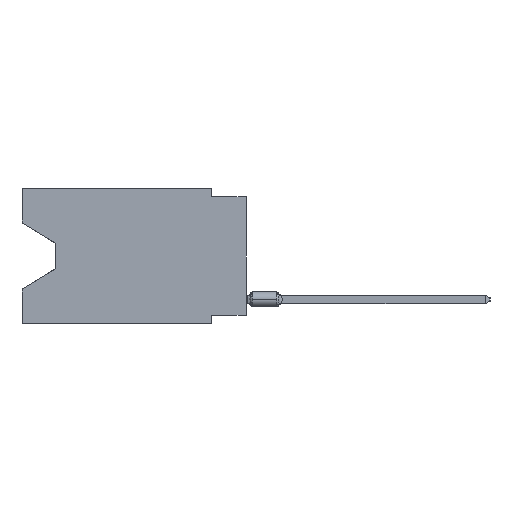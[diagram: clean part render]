
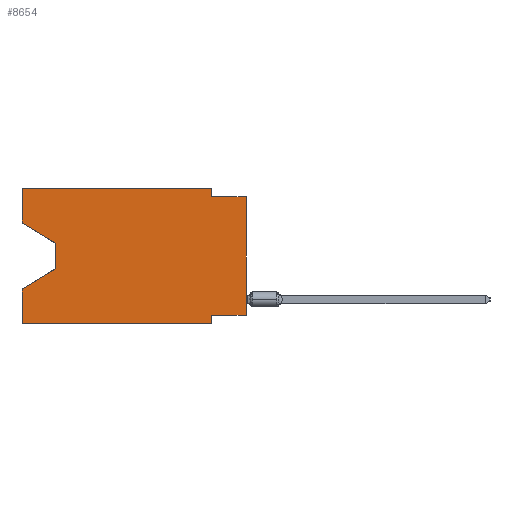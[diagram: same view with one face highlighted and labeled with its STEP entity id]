
A CAD part, left-side view. The second image highlights one B-rep face of the part: STEP entity #8654.
In plain terms, the highlighted planar face has unit normal (-1, 0, 0).
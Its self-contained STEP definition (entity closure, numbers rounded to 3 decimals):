
#57 = VECTOR ( 'NONE', #44217, 1000. ) ;
#443 = EDGE_CURVE ( 'NONE', #57725, #37738, #47207, .T. ) ;
#901 = CARTESIAN_POINT ( 'NONE',  ( 0., 2.54, 0. ) ) ;
#2306 = VERTEX_POINT ( 'NONE', #23278 ) ;
#3446 = DIRECTION ( 'NONE',  ( 0., 0., -1. ) ) ;
#3466 = EDGE_CURVE ( 'NONE', #30836, #67137, #64487, .T. ) ;
#4068 = DIRECTION ( 'NONE',  ( 0., 0., -1. ) ) ;
#4407 = ORIENTED_EDGE ( 'NONE', *, *, #6342, .F. ) ;
#4473 = VECTOR ( 'NONE', #26601, 1000. ) ;
#4868 = VERTEX_POINT ( 'NONE', #29654 ) ;
#5179 = CARTESIAN_POINT ( 'NONE',  ( 0., 0., -9.271 ) ) ;
#6342 = EDGE_CURVE ( 'NONE', #37738, #67137, #57201, .T. ) ;
#7583 = DIRECTION ( 'NONE',  ( 0., -0.855, -0.519 ) ) ;
#8487 = CARTESIAN_POINT ( 'NONE',  ( 0., 16.383, 0. ) ) ;
#8625 = ORIENTED_EDGE ( 'NONE', *, *, #38947, .T. ) ;
#8654 = ADVANCED_FACE ( 'NONE', ( #37394 ), #58468, .F. ) ;
#9928 = EDGE_CURVE ( 'NONE', #51150, #2306, #49291, .T. ) ;
#10958 = DIRECTION ( 'NONE',  ( 0., 1., 0. ) ) ;
#11368 = VECTOR ( 'NONE', #7583, 1000. ) ;
#14093 = CARTESIAN_POINT ( 'NONE',  ( 0., 16.383, -2.546 ) ) ;
#14217 = ORIENTED_EDGE ( 'NONE', *, *, #19808, .F. ) ;
#14324 = CARTESIAN_POINT ( 'NONE',  ( 0., 2.54, -9.906 ) ) ;
#14363 = VERTEX_POINT ( 'NONE', #35593 ) ;
#14561 = DIRECTION ( 'NONE',  ( 0., -1., 0. ) ) ;
#14882 = VERTEX_POINT ( 'NONE', #30804 ) ;
#15417 = LINE ( 'NONE', #27028, #56358 ) ;
#15752 = VECTOR ( 'NONE', #14561, 1000. ) ;
#17408 = VECTOR ( 'NONE', #53731, 1000. ) ;
#17792 = EDGE_CURVE ( 'NONE', #14882, #22995, #15417, .T. ) ;
#17950 = DIRECTION ( 'NONE',  ( 0., -1., 0. ) ) ;
#19123 = CARTESIAN_POINT ( 'NONE',  ( 0., 0., -0.635 ) ) ;
#19808 = EDGE_CURVE ( 'NONE', #14363, #22995, #36394, .T. ) ;
#20112 = ORIENTED_EDGE ( 'NONE', *, *, #9928, .F. ) ;
#20359 = CARTESIAN_POINT ( 'NONE',  ( 0., 2.54, -9.271 ) ) ;
#20832 = EDGE_CURVE ( 'NONE', #51150, #37796, #68490, .T. ) ;
#21746 = CARTESIAN_POINT ( 'NONE',  ( 0., 16.383, 0. ) ) ;
#22995 = VERTEX_POINT ( 'NONE', #52587 ) ;
#23278 = CARTESIAN_POINT ( 'NONE',  ( 0., 16.383, 0. ) ) ;
#26434 = CARTESIAN_POINT ( 'NONE',  ( 0., 0., 0. ) ) ;
#26601 = DIRECTION ( 'NONE',  ( 0., 0., 1. ) ) ;
#26919 = CARTESIAN_POINT ( 'NONE',  ( 0., 13.97, -4.013 ) ) ;
#27028 = CARTESIAN_POINT ( 'NONE',  ( 0., 13.97, -5.893 ) ) ;
#28239 = CARTESIAN_POINT ( 'NONE',  ( 0., 0., -0.635 ) ) ;
#28847 = LINE ( 'NONE', #50918, #31454 ) ;
#29654 = CARTESIAN_POINT ( 'NONE',  ( 0., 2.54, -9.906 ) ) ;
#30804 = CARTESIAN_POINT ( 'NONE',  ( 0., 13.97, -5.893 ) ) ;
#30836 = VERTEX_POINT ( 'NONE', #67482 ) ;
#31454 = VECTOR ( 'NONE', #17950, 1000. ) ;
#32580 = ORIENTED_EDGE ( 'NONE', *, *, #60871, .F. ) ;
#33423 = LINE ( 'NONE', #5179, #55248 ) ;
#34770 = ORIENTED_EDGE ( 'NONE', *, *, #69800, .T. ) ;
#35593 = CARTESIAN_POINT ( 'NONE',  ( 0., 16.383, -9.906 ) ) ;
#36394 = LINE ( 'NONE', #8487, #4473 ) ;
#36665 = CARTESIAN_POINT ( 'NONE',  ( 0., 16.383, 0. ) ) ;
#36751 = VECTOR ( 'NONE', #39782, 1000. ) ;
#37373 = LINE ( 'NONE', #36665, #15752 ) ;
#37394 = FACE_OUTER_BOUND ( 'NONE', #64142, .T. ) ;
#37506 = DIRECTION ( 'NONE',  ( 0., 0.855, -0.519 ) ) ;
#37738 = VERTEX_POINT ( 'NONE', #51568 ) ;
#37768 = ORIENTED_EDGE ( 'NONE', *, *, #46088, .F. ) ;
#37796 = VERTEX_POINT ( 'NONE', #48636 ) ;
#37979 = VECTOR ( 'NONE', #3446, 1000. ) ;
#38947 = EDGE_CURVE ( 'NONE', #14363, #4868, #28847, .T. ) ;
#39092 = VERTEX_POINT ( 'NONE', #20359 ) ;
#39782 = DIRECTION ( 'NONE',  ( 0., -1., 0. ) ) ;
#41856 = LINE ( 'NONE', #14324, #37979 ) ;
#43396 = ORIENTED_EDGE ( 'NONE', *, *, #20832, .T. ) ;
#44217 = DIRECTION ( 'NONE',  ( 0., 0., 1. ) ) ;
#46088 = EDGE_CURVE ( 'NONE', #39092, #4868, #41856, .T. ) ;
#47207 = LINE ( 'NONE', #48628, #17408 ) ;
#47704 = CARTESIAN_POINT ( 'NONE',  ( 0., 16.383, -2.546 ) ) ;
#47913 = DIRECTION ( 'NONE',  ( 1., 0., 0. ) ) ;
#48110 = ORIENTED_EDGE ( 'NONE', *, *, #443, .F. ) ;
#48628 = CARTESIAN_POINT ( 'NONE',  ( 0., 2.54, 0. ) ) ;
#48636 = CARTESIAN_POINT ( 'NONE',  ( 0., 13.97, -4.013 ) ) ;
#49291 = LINE ( 'NONE', #21746, #57 ) ;
#50918 = CARTESIAN_POINT ( 'NONE',  ( 0., 16.383, -9.906 ) ) ;
#50968 = ORIENTED_EDGE ( 'NONE', *, *, #3466, .T. ) ;
#51150 = VERTEX_POINT ( 'NONE', #47704 ) ;
#51568 = CARTESIAN_POINT ( 'NONE',  ( 0., 2.54, -0.635 ) ) ;
#52587 = CARTESIAN_POINT ( 'NONE',  ( 0., 16.383, -7.36 ) ) ;
#53720 = CARTESIAN_POINT ( 'NONE',  ( 0., 16.383, 0. ) ) ;
#53731 = DIRECTION ( 'NONE',  ( 0., 0., -1. ) ) ;
#54083 = DIRECTION ( 'NONE',  ( 0., 0., -1. ) ) ;
#55248 = VECTOR ( 'NONE', #10958, 1000. ) ;
#56358 = VECTOR ( 'NONE', #37506, 1000. ) ;
#56914 = VECTOR ( 'NONE', #54083, 1000. ) ;
#57106 = EDGE_CURVE ( 'NONE', #2306, #57725, #37373, .T. ) ;
#57201 = LINE ( 'NONE', #19123, #36751 ) ;
#57725 = VERTEX_POINT ( 'NONE', #901 ) ;
#58468 = PLANE ( 'NONE',  #68232 ) ;
#58615 = VECTOR ( 'NONE', #59420, 1000. ) ;
#59420 = DIRECTION ( 'NONE',  ( 0., 0., 1. ) ) ;
#60871 = EDGE_CURVE ( 'NONE', #30836, #39092, #33423, .T. ) ;
#64074 = ORIENTED_EDGE ( 'NONE', *, *, #17792, .T. ) ;
#64142 = EDGE_LOOP ( 'NONE', ( #43396, #34770, #64074, #14217, #8625, #37768, #32580, #50968, #4407, #48110, #65379, #20112 ) ) ;
#64487 = LINE ( 'NONE', #26434, #58615 ) ;
#65334 = LINE ( 'NONE', #26919, #56914 ) ;
#65379 = ORIENTED_EDGE ( 'NONE', *, *, #57106, .F. ) ;
#67137 = VERTEX_POINT ( 'NONE', #28239 ) ;
#67482 = CARTESIAN_POINT ( 'NONE',  ( 0., 0., -9.271 ) ) ;
#68232 = AXIS2_PLACEMENT_3D ( 'NONE', #53720, #47913, #4068 ) ;
#68490 = LINE ( 'NONE', #14093, #11368 ) ;
#69800 = EDGE_CURVE ( 'NONE', #37796, #14882, #65334, .T. ) ;
